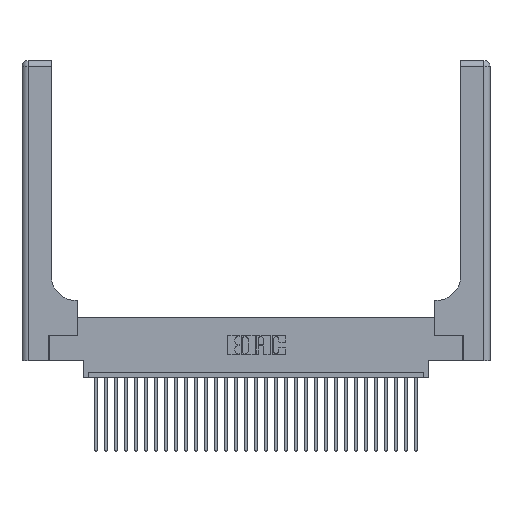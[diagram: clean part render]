
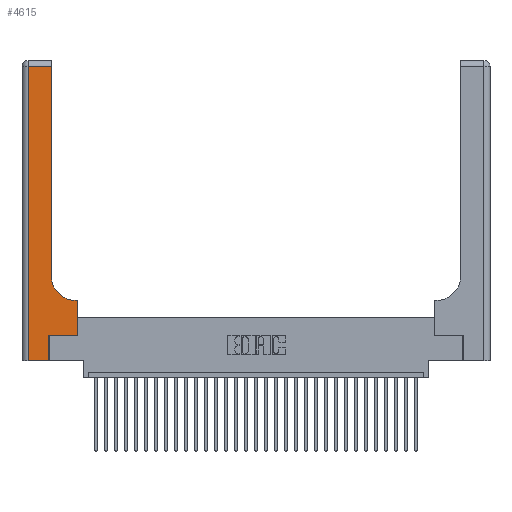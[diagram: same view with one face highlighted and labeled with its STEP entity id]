
A CAD part, top view. The second image highlights one B-rep face of the part: STEP entity #4615.
In plain terms, the highlighted planar face has unit normal (0, 0, 1).
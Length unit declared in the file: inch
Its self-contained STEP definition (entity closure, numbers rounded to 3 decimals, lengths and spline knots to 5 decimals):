
#317 = VERTEX_POINT ( 'NONE', #6716 ) ;
#405 = EDGE_CURVE ( 'NONE', #21446, #20029, #27459, .T. ) ;
#444 = VECTOR ( 'NONE', #26753, 39.37008 ) ;
#1066 = LINE ( 'NONE', #27815, #20816 ) ;
#1265 = CARTESIAN_POINT ( 'NONE',  ( 0., 3., 0.37 ) ) ;
#1361 = DIRECTION ( 'NONE',  ( 0., 0., -1. ) ) ;
#1745 = VERTEX_POINT ( 'NONE', #3750 ) ;
#3203 = LINE ( 'NONE', #17199, #6217 ) ;
#3750 = CARTESIAN_POINT ( 'NONE',  ( 0.5585, 0.6, 0.37 ) ) ;
#3806 = DIRECTION ( 'NONE',  ( -1., 0., 0. ) ) ;
#4298 = DIRECTION ( 'NONE',  ( 0., -1., 0. ) ) ;
#4322 = VECTOR ( 'NONE', #14089, 39.37008 ) ;
#4615 = ADVANCED_FACE ( 'NONE', ( #29814 ), #8968, .F. ) ;
#4829 = CARTESIAN_POINT ( 'NONE',  ( 0.269, 0., 0.37 ) ) ;
#4881 = CARTESIAN_POINT ( 'NONE',  ( 0.269, 0.25, 0.37 ) ) ;
#5679 = CARTESIAN_POINT ( 'NONE',  ( 0.06, 2.94, 0.37 ) ) ;
#5774 = EDGE_CURVE ( 'NONE', #27345, #1745, #1066, .T. ) ;
#6217 = VECTOR ( 'NONE', #17099, 39.37008 ) ;
#6716 = CARTESIAN_POINT ( 'NONE',  ( 0.269, 0.25, 0.37 ) ) ;
#6778 = ORIENTED_EDGE ( 'NONE', *, *, #13545, .T. ) ;
#6900 = VERTEX_POINT ( 'NONE', #21772 ) ;
#7012 = LINE ( 'NONE', #11535, #19175 ) ;
#7476 = VECTOR ( 'NONE', #20767, 39.37008 ) ;
#8244 = EDGE_CURVE ( 'NONE', #1745, #9001, #16830, .T. ) ;
#8968 = PLANE ( 'NONE',  #28367 ) ;
#9001 = VERTEX_POINT ( 'NONE', #13289 ) ;
#9014 = CARTESIAN_POINT ( 'NONE',  ( 0.2915, 3., 0.37 ) ) ;
#9201 = ORIENTED_EDGE ( 'NONE', *, *, #16295, .T. ) ;
#9721 = CARTESIAN_POINT ( 'NONE',  ( 0.2915, 2.94, 0.37 ) ) ;
#10702 = LINE ( 'NONE', #4881, #28158 ) ;
#10882 = VERTEX_POINT ( 'NONE', #5679 ) ;
#10977 = EDGE_CURVE ( 'NONE', #9001, #21446, #18985, .T. ) ;
#11324 = ORIENTED_EDGE ( 'NONE', *, *, #8244, .T. ) ;
#11483 = VERTEX_POINT ( 'NONE', #16691 ) ;
#11499 = ORIENTED_EDGE ( 'NONE', *, *, #19207, .T. ) ;
#11535 = CARTESIAN_POINT ( 'NONE',  ( 0.06, 3., 0.37 ) ) ;
#11804 = EDGE_CURVE ( 'NONE', #6900, #11483, #3203, .T. ) ;
#13212 = ORIENTED_EDGE ( 'NONE', *, *, #21540, .T. ) ;
#13289 = CARTESIAN_POINT ( 'NONE',  ( 0.5415, 0.6, 0.37 ) ) ;
#13545 = EDGE_CURVE ( 'NONE', #11483, #317, #19784, .T. ) ;
#13910 = LINE ( 'NONE', #20567, #7476 ) ;
#14089 = DIRECTION ( 'NONE',  ( 0., 1., 0. ) ) ;
#15471 = ORIENTED_EDGE ( 'NONE', *, *, #10977, .T. ) ;
#16295 = EDGE_CURVE ( 'NONE', #20029, #10882, #13910, .T. ) ;
#16691 = CARTESIAN_POINT ( 'NONE',  ( 0.269, 0., 0.37 ) ) ;
#16830 = LINE ( 'NONE', #23742, #22159 ) ;
#17099 = DIRECTION ( 'NONE',  ( 1., 0., 0. ) ) ;
#17199 = CARTESIAN_POINT ( 'NONE',  ( 0., 0., 0.37 ) ) ;
#18985 = CIRCLE ( 'NONE', #20106, 0.25 ) ;
#19019 = CARTESIAN_POINT ( 'NONE',  ( 0.5585, 0.25, 0.37 ) ) ;
#19175 = VECTOR ( 'NONE', #4298, 39.37008 ) ;
#19207 = EDGE_CURVE ( 'NONE', #10882, #6900, #7012, .T. ) ;
#19515 = DIRECTION ( 'NONE',  ( 1., 0., 0. ) ) ;
#19723 = CARTESIAN_POINT ( 'NONE',  ( 0.2915, 0.85, 0.37 ) ) ;
#19784 = LINE ( 'NONE', #4829, #444 ) ;
#20029 = VERTEX_POINT ( 'NONE', #9721 ) ;
#20043 = CARTESIAN_POINT ( 'NONE',  ( 0.5415, 0.85, 0.37 ) ) ;
#20106 = AXIS2_PLACEMENT_3D ( 'NONE', #20043, #26425, #21020 ) ;
#20203 = DIRECTION ( 'NONE',  ( 0., 1., 0. ) ) ;
#20567 = CARTESIAN_POINT ( 'NONE',  ( 0., 2.94, 0.37 ) ) ;
#20767 = DIRECTION ( 'NONE',  ( -1., 0., 0. ) ) ;
#20816 = VECTOR ( 'NONE', #20203, 39.37008 ) ;
#21020 = DIRECTION ( 'NONE',  ( 1., 0., 0. ) ) ;
#21446 = VERTEX_POINT ( 'NONE', #19723 ) ;
#21540 = EDGE_CURVE ( 'NONE', #317, #27345, #10702, .T. ) ;
#21772 = CARTESIAN_POINT ( 'NONE',  ( 0.06, 0., 0.37 ) ) ;
#22159 = VECTOR ( 'NONE', #25949, 39.37008 ) ;
#23742 = CARTESIAN_POINT ( 'NONE',  ( 0.2915, 0.6, 0.37 ) ) ;
#24548 = ORIENTED_EDGE ( 'NONE', *, *, #5774, .T. ) ;
#25446 = ORIENTED_EDGE ( 'NONE', *, *, #405, .T. ) ;
#25949 = DIRECTION ( 'NONE',  ( -1., 0., 0. ) ) ;
#26425 = DIRECTION ( 'NONE',  ( 0., 0., -1. ) ) ;
#26753 = DIRECTION ( 'NONE',  ( 0., 1., 0. ) ) ;
#26933 = EDGE_LOOP ( 'NONE', ( #25446, #9201, #11499, #29850, #6778, #13212, #24548, #11324, #15471 ) ) ;
#27345 = VERTEX_POINT ( 'NONE', #19019 ) ;
#27459 = LINE ( 'NONE', #9014, #4322 ) ;
#27815 = CARTESIAN_POINT ( 'NONE',  ( 0.5585, 0.25, 0.37 ) ) ;
#28158 = VECTOR ( 'NONE', #19515, 39.37008 ) ;
#28367 = AXIS2_PLACEMENT_3D ( 'NONE', #1265, #1361, #3806 ) ;
#29814 = FACE_OUTER_BOUND ( 'NONE', #26933, .T. ) ;
#29850 = ORIENTED_EDGE ( 'NONE', *, *, #11804, .T. ) ;
